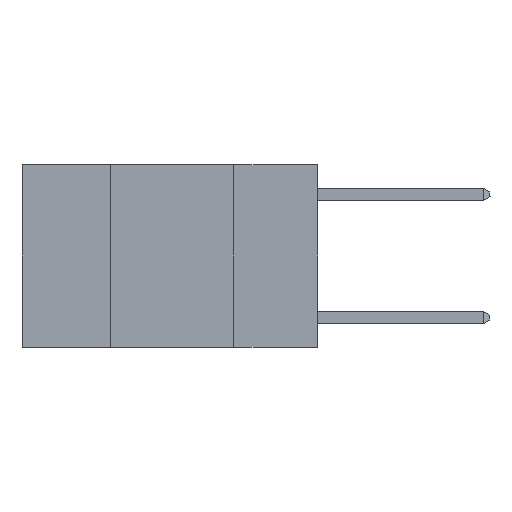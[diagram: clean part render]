
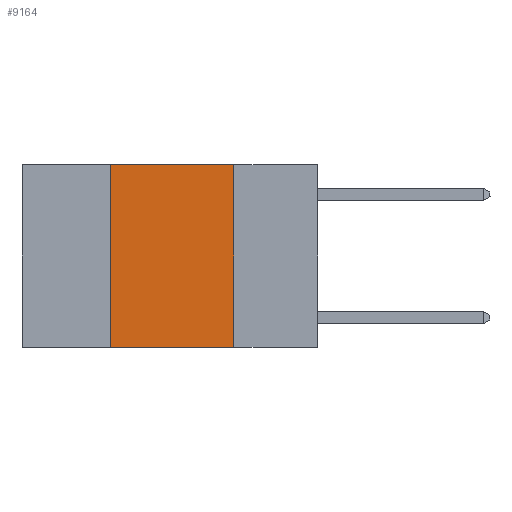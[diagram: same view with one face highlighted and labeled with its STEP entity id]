
A CAD part, left-side view. The second image highlights one B-rep face of the part: STEP entity #9164.
In plain terms, the highlighted planar face has unit normal (-1, 0, 0).
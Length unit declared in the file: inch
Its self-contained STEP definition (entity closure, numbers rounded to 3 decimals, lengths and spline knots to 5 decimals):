
#326 = EDGE_LOOP ( 'NONE', ( #3455, #673, #1267, #10503 ) ) ;
#673 = ORIENTED_EDGE ( 'NONE', *, *, #6943, .F. ) ;
#873 = AXIS2_PLACEMENT_3D ( 'NONE', #8491, #2997, #9405 ) ;
#1267 = ORIENTED_EDGE ( 'NONE', *, *, #9647, .F. ) ;
#1540 = CARTESIAN_POINT ( 'NONE',  ( 0., 0.17, -0.37 ) ) ;
#2064 = PLANE ( 'NONE',  #873 ) ;
#2092 = VECTOR ( 'NONE', #3557, 39.37008 ) ;
#2667 = CARTESIAN_POINT ( 'NONE',  ( 0., 0.6, 0. ) ) ;
#2726 = VECTOR ( 'NONE', #8145, 39.37008 ) ;
#2997 = DIRECTION ( 'NONE',  ( 1., 0., 0. ) ) ;
#3455 = ORIENTED_EDGE ( 'NONE', *, *, #4925, .F. ) ;
#3516 = DIRECTION ( 'NONE',  ( 0., -1., 0. ) ) ;
#3557 = DIRECTION ( 'NONE',  ( 0., 0., 1. ) ) ;
#3814 = FACE_OUTER_BOUND ( 'NONE', #326, .T. ) ;
#3929 = CARTESIAN_POINT ( 'NONE',  ( 0., 0.42, -0.37 ) ) ;
#4445 = CARTESIAN_POINT ( 'NONE',  ( 0., 0.6, -0.37 ) ) ;
#4547 = CARTESIAN_POINT ( 'NONE',  ( 0., 0.42, 0. ) ) ;
#4560 = VECTOR ( 'NONE', #3516, 39.37008 ) ;
#4925 = EDGE_CURVE ( 'NONE', #8370, #9488, #6177, .T. ) ;
#5910 = VERTEX_POINT ( 'NONE', #3929 ) ;
#6177 = LINE ( 'NONE', #6366, #8288 ) ;
#6366 = CARTESIAN_POINT ( 'NONE',  ( 0., 0.17, 0. ) ) ;
#6626 = CARTESIAN_POINT ( 'NONE',  ( 0., 0.17, 0. ) ) ;
#6703 = LINE ( 'NONE', #9973, #2092 ) ;
#6943 = EDGE_CURVE ( 'NONE', #8881, #8370, #9752, .T. ) ;
#8145 = DIRECTION ( 'NONE',  ( 0., -1., 0. ) ) ;
#8179 = DIRECTION ( 'NONE',  ( 0., 0., -1. ) ) ;
#8288 = VECTOR ( 'NONE', #8179, 39.37008 ) ;
#8370 = VERTEX_POINT ( 'NONE', #6626 ) ;
#8491 = CARTESIAN_POINT ( 'NONE',  ( 0., 0.6, 0. ) ) ;
#8881 = VERTEX_POINT ( 'NONE', #4547 ) ;
#9164 = ADVANCED_FACE ( 'NONE', ( #3814 ), #2064, .F. ) ;
#9405 = DIRECTION ( 'NONE',  ( 0., 0., -1. ) ) ;
#9488 = VERTEX_POINT ( 'NONE', #1540 ) ;
#9610 = EDGE_CURVE ( 'NONE', #5910, #9488, #11942, .T. ) ;
#9647 = EDGE_CURVE ( 'NONE', #5910, #8881, #6703, .T. ) ;
#9752 = LINE ( 'NONE', #2667, #2726 ) ;
#9973 = CARTESIAN_POINT ( 'NONE',  ( 0., 0.42, 0. ) ) ;
#10503 = ORIENTED_EDGE ( 'NONE', *, *, #9610, .T. ) ;
#11942 = LINE ( 'NONE', #4445, #4560 ) ;
